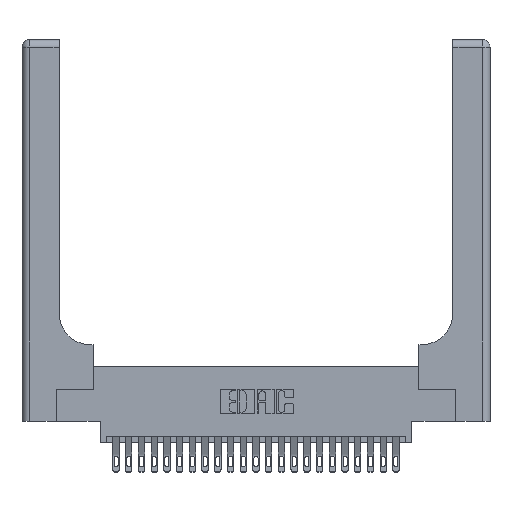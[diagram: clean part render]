
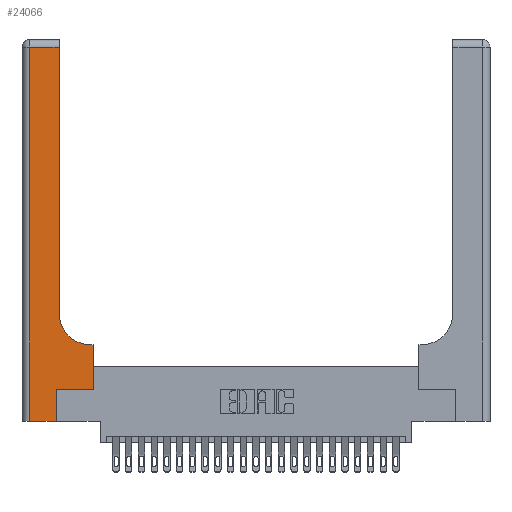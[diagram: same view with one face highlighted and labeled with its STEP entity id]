
A CAD part, top view. The second image highlights one B-rep face of the part: STEP entity #24066.
In plain terms, the highlighted planar face has unit normal (0, 0, 1).
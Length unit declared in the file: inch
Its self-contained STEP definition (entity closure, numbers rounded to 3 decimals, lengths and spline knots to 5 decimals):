
#148 = CARTESIAN_POINT ( 'NONE',  ( 0.06, 0., 0.37 ) ) ;
#292 = FACE_OUTER_BOUND ( 'NONE', #713, .T. ) ;
#415 = CARTESIAN_POINT ( 'NONE',  ( 0., 0., 0.37 ) ) ;
#693 = ORIENTED_EDGE ( 'NONE', *, *, #24120, .T. ) ;
#701 = LINE ( 'NONE', #415, #5544 ) ;
#713 = EDGE_LOOP ( 'NONE', ( #4911, #15271, #25400, #9786, #693, #25489, #15575, #20606, #7241 ) ) ;
#962 = CARTESIAN_POINT ( 'NONE',  ( 0.269, 0.25, 0.37 ) ) ;
#1060 = VECTOR ( 'NONE', #14019, 39.37008 ) ;
#1262 = CARTESIAN_POINT ( 'NONE',  ( 0.2915, 2.94, 0.37 ) ) ;
#1745 = CARTESIAN_POINT ( 'NONE',  ( 0.5585, 0.25, 0.37 ) ) ;
#1980 = EDGE_CURVE ( 'NONE', #4040, #23081, #4783, .T. ) ;
#3045 = CARTESIAN_POINT ( 'NONE',  ( 0.06, 2.94, 0.37 ) ) ;
#3885 = DIRECTION ( 'NONE',  ( 0., 0., -1. ) ) ;
#4040 = VERTEX_POINT ( 'NONE', #25806 ) ;
#4783 = LINE ( 'NONE', #962, #26249 ) ;
#4854 = CIRCLE ( 'NONE', #7945, 0.25 ) ;
#4911 = ORIENTED_EDGE ( 'NONE', *, *, #9242, .T. ) ;
#5145 = VECTOR ( 'NONE', #15717, 39.37008 ) ;
#5373 = CARTESIAN_POINT ( 'NONE',  ( 0., 3., 0.37 ) ) ;
#5544 = VECTOR ( 'NONE', #22881, 39.37008 ) ;
#6115 = VECTOR ( 'NONE', #23577, 39.37008 ) ;
#6784 = VERTEX_POINT ( 'NONE', #15176 ) ;
#7241 = ORIENTED_EDGE ( 'NONE', *, *, #14902, .T. ) ;
#7375 = CARTESIAN_POINT ( 'NONE',  ( 0.5585, 0.25, 0.37 ) ) ;
#7430 = DIRECTION ( 'NONE',  ( -1., 0., 0. ) ) ;
#7562 = DIRECTION ( 'NONE',  ( -1., 0., 0. ) ) ;
#7577 = CARTESIAN_POINT ( 'NONE',  ( 0.269, 0., 0.37 ) ) ;
#7920 = DIRECTION ( 'NONE',  ( 0., -1., 0. ) ) ;
#7945 = AXIS2_PLACEMENT_3D ( 'NONE', #16220, #3885, #18247 ) ;
#8903 = VERTEX_POINT ( 'NONE', #3045 ) ;
#9161 = EDGE_CURVE ( 'NONE', #8903, #11112, #11963, .T. ) ;
#9242 = EDGE_CURVE ( 'NONE', #9392, #18088, #26060, .T. ) ;
#9382 = VECTOR ( 'NONE', #20490, 39.37008 ) ;
#9392 = VERTEX_POINT ( 'NONE', #20915 ) ;
#9403 = EDGE_CURVE ( 'NONE', #11112, #14867, #701, .T. ) ;
#9475 = CARTESIAN_POINT ( 'NONE',  ( 0.269, 0., 0.37 ) ) ;
#9601 = AXIS2_PLACEMENT_3D ( 'NONE', #5373, #19687, #7430 ) ;
#9786 = ORIENTED_EDGE ( 'NONE', *, *, #9403, .T. ) ;
#10570 = LINE ( 'NONE', #9475, #5145 ) ;
#11112 = VERTEX_POINT ( 'NONE', #148 ) ;
#11963 = LINE ( 'NONE', #26037, #22117 ) ;
#12747 = VERTEX_POINT ( 'NONE', #14777 ) ;
#13650 = EDGE_CURVE ( 'NONE', #18088, #8903, #22732, .T. ) ;
#14019 = DIRECTION ( 'NONE',  ( -1., 0., 0. ) ) ;
#14777 = CARTESIAN_POINT ( 'NONE',  ( 0.5585, 0.6, 0.37 ) ) ;
#14867 = VERTEX_POINT ( 'NONE', #7577 ) ;
#14902 = EDGE_CURVE ( 'NONE', #6784, #9392, #4854, .T. ) ;
#15055 = VECTOR ( 'NONE', #7562, 39.37008 ) ;
#15176 = CARTESIAN_POINT ( 'NONE',  ( 0.5415, 0.6, 0.37 ) ) ;
#15271 = ORIENTED_EDGE ( 'NONE', *, *, #13650, .T. ) ;
#15359 = DIRECTION ( 'NONE',  ( 1., 0., 0. ) ) ;
#15387 = EDGE_CURVE ( 'NONE', #23081, #12747, #16403, .T. ) ;
#15575 = ORIENTED_EDGE ( 'NONE', *, *, #15387, .T. ) ;
#15717 = DIRECTION ( 'NONE',  ( 0., 1., 0. ) ) ;
#16220 = CARTESIAN_POINT ( 'NONE',  ( 0.5415, 0.85, 0.37 ) ) ;
#16403 = LINE ( 'NONE', #7375, #6115 ) ;
#18088 = VERTEX_POINT ( 'NONE', #1262 ) ;
#18247 = DIRECTION ( 'NONE',  ( 1., 0., 0. ) ) ;
#19687 = DIRECTION ( 'NONE',  ( 0., 0., -1. ) ) ;
#20490 = DIRECTION ( 'NONE',  ( 0., 1., 0. ) ) ;
#20606 = ORIENTED_EDGE ( 'NONE', *, *, #25314, .T. ) ;
#20915 = CARTESIAN_POINT ( 'NONE',  ( 0.2915, 0.85, 0.37 ) ) ;
#21716 = CARTESIAN_POINT ( 'NONE',  ( 0.2915, 3., 0.37 ) ) ;
#21790 = CARTESIAN_POINT ( 'NONE',  ( 0.2915, 0.6, 0.37 ) ) ;
#22117 = VECTOR ( 'NONE', #7920, 39.37008 ) ;
#22732 = LINE ( 'NONE', #23975, #1060 ) ;
#22881 = DIRECTION ( 'NONE',  ( 1., 0., 0. ) ) ;
#23081 = VERTEX_POINT ( 'NONE', #1745 ) ;
#23577 = DIRECTION ( 'NONE',  ( 0., 1., 0. ) ) ;
#23975 = CARTESIAN_POINT ( 'NONE',  ( 0., 2.94, 0.37 ) ) ;
#24066 = ADVANCED_FACE ( 'NONE', ( #292 ), #25508, .F. ) ;
#24120 = EDGE_CURVE ( 'NONE', #14867, #4040, #10570, .T. ) ;
#25314 = EDGE_CURVE ( 'NONE', #12747, #6784, #25623, .T. ) ;
#25400 = ORIENTED_EDGE ( 'NONE', *, *, #9161, .T. ) ;
#25489 = ORIENTED_EDGE ( 'NONE', *, *, #1980, .T. ) ;
#25508 = PLANE ( 'NONE',  #9601 ) ;
#25623 = LINE ( 'NONE', #21790, #15055 ) ;
#25806 = CARTESIAN_POINT ( 'NONE',  ( 0.269, 0.25, 0.37 ) ) ;
#26037 = CARTESIAN_POINT ( 'NONE',  ( 0.06, 3., 0.37 ) ) ;
#26060 = LINE ( 'NONE', #21716, #9382 ) ;
#26249 = VECTOR ( 'NONE', #15359, 39.37008 ) ;
